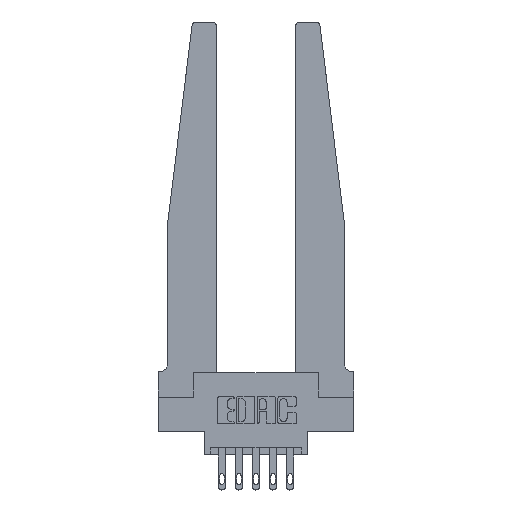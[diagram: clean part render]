
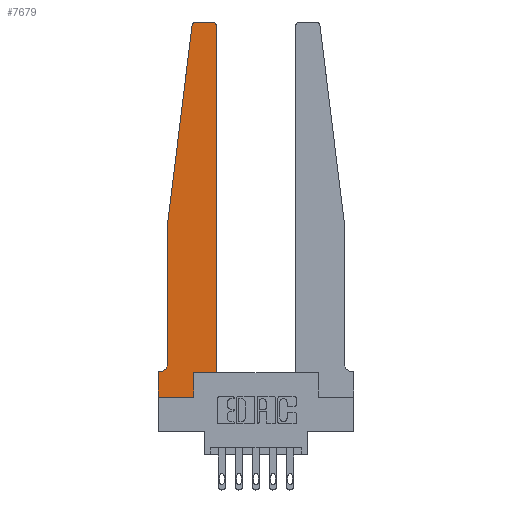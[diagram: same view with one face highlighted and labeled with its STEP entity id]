
A CAD part, top view. The second image highlights one B-rep face of the part: STEP entity #7679.
In plain terms, the highlighted planar face has unit normal (0, 0, 1).
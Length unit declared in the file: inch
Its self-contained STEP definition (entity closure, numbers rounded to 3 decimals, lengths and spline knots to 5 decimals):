
#95 = EDGE_CURVE ( 'NONE', #11984, #3041, #4110, .T. ) ;
#218 = LINE ( 'NONE', #8400, #6895 ) ;
#264 = EDGE_CURVE ( 'NONE', #709, #2910, #1304, .T. ) ;
#265 = ORIENTED_EDGE ( 'NONE', *, *, #1896, .T. ) ;
#308 = LINE ( 'NONE', #11631, #12853 ) ;
#404 = VECTOR ( 'NONE', #2704, 39.37008 ) ;
#709 = VERTEX_POINT ( 'NONE', #11188 ) ;
#835 = VERTEX_POINT ( 'NONE', #3044 ) ;
#937 = VERTEX_POINT ( 'NONE', #10650 ) ;
#1180 = DIRECTION ( 'NONE',  ( 0., 0., 1. ) ) ;
#1304 = LINE ( 'NONE', #5456, #3868 ) ;
#1306 = CARTESIAN_POINT ( 'NONE',  ( 0.425, 0.18, 0.37 ) ) ;
#1323 = DIRECTION ( 'NONE',  ( 1., 0., 0. ) ) ;
#1504 = CIRCLE ( 'NONE', #7797, 0.03 ) ;
#1692 = EDGE_CURVE ( 'NONE', #3041, #10198, #8626, .T. ) ;
#1896 = EDGE_CURVE ( 'NONE', #835, #11175, #308, .T. ) ;
#1993 = CARTESIAN_POINT ( 'NONE',  ( 0.065, 0.2375, 0.37 ) ) ;
#2194 = EDGE_CURVE ( 'NONE', #10724, #7500, #1504, .T. ) ;
#2220 = CARTESIAN_POINT ( 'NONE',  ( 0., 0.1875, 0.37 ) ) ;
#2389 = DIRECTION ( 'NONE',  ( 1., 0., 0. ) ) ;
#2543 = CARTESIAN_POINT ( 'NONE',  ( 0.2605, 0., 0.37 ) ) ;
#2657 = CARTESIAN_POINT ( 'NONE',  ( 0.395, 2.72, 0.37 ) ) ;
#2704 = DIRECTION ( 'NONE',  ( -0.122, -0.992, 0. ) ) ;
#2910 = VERTEX_POINT ( 'NONE', #2937 ) ;
#2917 = DIRECTION ( 'NONE',  ( 0., 0., 1. ) ) ;
#2937 = CARTESIAN_POINT ( 'NONE',  ( 0.425, 0.18, 0.37 ) ) ;
#3041 = VERTEX_POINT ( 'NONE', #1993 ) ;
#3044 = CARTESIAN_POINT ( 'NONE',  ( 0., 0., 0.37 ) ) ;
#3350 = LINE ( 'NONE', #1306, #13443 ) ;
#3492 = DIRECTION ( 'NONE',  ( 1., 0., 0. ) ) ;
#3603 = VECTOR ( 'NONE', #12842, 39.37008 ) ;
#3653 = ORIENTED_EDGE ( 'NONE', *, *, #1692, .T. ) ;
#3741 = CARTESIAN_POINT ( 'NONE',  ( 0.065, 0.1875, 0.37 ) ) ;
#3868 = VECTOR ( 'NONE', #3492, 39.37008 ) ;
#4110 = LINE ( 'NONE', #9196, #8848 ) ;
#4134 = DIRECTION ( 'NONE',  ( 0., -1., 0. ) ) ;
#4349 = ORIENTED_EDGE ( 'NONE', *, *, #2194, .T. ) ;
#4383 = CARTESIAN_POINT ( 'NONE',  ( 0.27653, 2.75, 0.37 ) ) ;
#4401 = ORIENTED_EDGE ( 'NONE', *, *, #12631, .T. ) ;
#5456 = CARTESIAN_POINT ( 'NONE',  ( 0.425, 0.18, 0.37 ) ) ;
#5982 = DIRECTION ( 'NONE',  ( 1., 0., 0. ) ) ;
#6377 = ORIENTED_EDGE ( 'NONE', *, *, #11007, .T. ) ;
#6508 = DIRECTION ( 'NONE',  ( 0., 1., 0. ) ) ;
#6750 = CARTESIAN_POINT ( 'NONE',  ( 0.015, 0.2375, 0.37 ) ) ;
#6859 = LINE ( 'NONE', #3741, #10986 ) ;
#6895 = VECTOR ( 'NONE', #6508, 39.37008 ) ;
#7035 = ORIENTED_EDGE ( 'NONE', *, *, #95, .T. ) ;
#7053 = CARTESIAN_POINT ( 'NONE',  ( 0.27653, 2.72, 0.37 ) ) ;
#7311 = EDGE_CURVE ( 'NONE', #11368, #11984, #9848, .T. ) ;
#7500 = VERTEX_POINT ( 'NONE', #12445 ) ;
#7519 = PLANE ( 'NONE',  #12578 ) ;
#7618 = EDGE_CURVE ( 'NONE', #11175, #709, #218, .T. ) ;
#7679 = ADVANCED_FACE ( 'NONE', ( #12506 ), #7519, .T. ) ;
#7797 = AXIS2_PLACEMENT_3D ( 'NONE', #2657, #2917, #5982 ) ;
#7801 = ORIENTED_EDGE ( 'NONE', *, *, #9173, .T. ) ;
#7867 = CARTESIAN_POINT ( 'NONE',  ( 0.065, 1.25, 0.37 ) ) ;
#7977 = CARTESIAN_POINT ( 'NONE',  ( 0.425, 2.72, 0.37 ) ) ;
#8102 = VERTEX_POINT ( 'NONE', #4383 ) ;
#8377 = CARTESIAN_POINT ( 'NONE',  ( 0.065, 1.25, 0.37 ) ) ;
#8400 = CARTESIAN_POINT ( 'NONE',  ( 0.2605, 0.18, 0.37 ) ) ;
#8626 = CIRCLE ( 'NONE', #8835, 0.05 ) ;
#8835 = AXIS2_PLACEMENT_3D ( 'NONE', #6750, #10897, #9947 ) ;
#8848 = VECTOR ( 'NONE', #10155, 39.37008 ) ;
#9066 = ORIENTED_EDGE ( 'NONE', *, *, #264, .T. ) ;
#9102 = DIRECTION ( 'NONE',  ( 1., 0., 0. ) ) ;
#9173 = EDGE_CURVE ( 'NONE', #7500, #8102, #9885, .T. ) ;
#9196 = CARTESIAN_POINT ( 'NONE',  ( 0.065, 1.25, 0.37 ) ) ;
#9295 = CARTESIAN_POINT ( 'NONE',  ( 0., 0., 0.37 ) ) ;
#9319 = DIRECTION ( 'NONE',  ( 0., 0., 1. ) ) ;
#9496 = VECTOR ( 'NONE', #4134, 39.37008 ) ;
#9707 = EDGE_CURVE ( 'NONE', #10198, #937, #6859, .T. ) ;
#9848 = LINE ( 'NONE', #7867, #404 ) ;
#9885 = LINE ( 'NONE', #11940, #3603 ) ;
#9947 = DIRECTION ( 'NONE',  ( -1., 0., 0. ) ) ;
#10026 = ORIENTED_EDGE ( 'NONE', *, *, #9707, .T. ) ;
#10155 = DIRECTION ( 'NONE',  ( 0., -1., 0. ) ) ;
#10198 = VERTEX_POINT ( 'NONE', #12927 ) ;
#10422 = EDGE_CURVE ( 'NONE', #937, #835, #11329, .T. ) ;
#10650 = CARTESIAN_POINT ( 'NONE',  ( 0., 0.1875, 0.37 ) ) ;
#10724 = VERTEX_POINT ( 'NONE', #7977 ) ;
#10799 = AXIS2_PLACEMENT_3D ( 'NONE', #7053, #9319, #9102 ) ;
#10897 = DIRECTION ( 'NONE',  ( 0., 0., -1. ) ) ;
#10986 = VECTOR ( 'NONE', #11018, 39.37008 ) ;
#11007 = EDGE_CURVE ( 'NONE', #2910, #10724, #3350, .T. ) ;
#11018 = DIRECTION ( 'NONE',  ( -1., 0., 0. ) ) ;
#11043 = ORIENTED_EDGE ( 'NONE', *, *, #7311, .T. ) ;
#11175 = VERTEX_POINT ( 'NONE', #2543 ) ;
#11188 = CARTESIAN_POINT ( 'NONE',  ( 0.2605, 0.18, 0.37 ) ) ;
#11329 = LINE ( 'NONE', #9295, #9496 ) ;
#11368 = VERTEX_POINT ( 'NONE', #11773 ) ;
#11431 = ORIENTED_EDGE ( 'NONE', *, *, #10422, .T. ) ;
#11517 = DIRECTION ( 'NONE',  ( 0., 1., 0. ) ) ;
#11631 = CARTESIAN_POINT ( 'NONE',  ( 0., 0., 0.37 ) ) ;
#11773 = CARTESIAN_POINT ( 'NONE',  ( 0.24675, 2.72367, 0.37 ) ) ;
#11940 = CARTESIAN_POINT ( 'NONE',  ( 0.25, 2.75, 0.37 ) ) ;
#11984 = VERTEX_POINT ( 'NONE', #8377 ) ;
#12442 = EDGE_LOOP ( 'NONE', ( #7801, #4401, #11043, #7035, #3653, #10026, #11431, #265, #12514, #9066, #6377, #4349 ) ) ;
#12445 = CARTESIAN_POINT ( 'NONE',  ( 0.395, 2.75, 0.37 ) ) ;
#12506 = FACE_OUTER_BOUND ( 'NONE', #12442, .T. ) ;
#12514 = ORIENTED_EDGE ( 'NONE', *, *, #7618, .T. ) ;
#12578 = AXIS2_PLACEMENT_3D ( 'NONE', #2220, #1180, #1323 ) ;
#12631 = EDGE_CURVE ( 'NONE', #8102, #11368, #13223, .T. ) ;
#12842 = DIRECTION ( 'NONE',  ( -1., 0., 0. ) ) ;
#12853 = VECTOR ( 'NONE', #2389, 39.37008 ) ;
#12927 = CARTESIAN_POINT ( 'NONE',  ( 0.015, 0.1875, 0.37 ) ) ;
#13223 = CIRCLE ( 'NONE', #10799, 0.03 ) ;
#13443 = VECTOR ( 'NONE', #11517, 39.37008 ) ;
